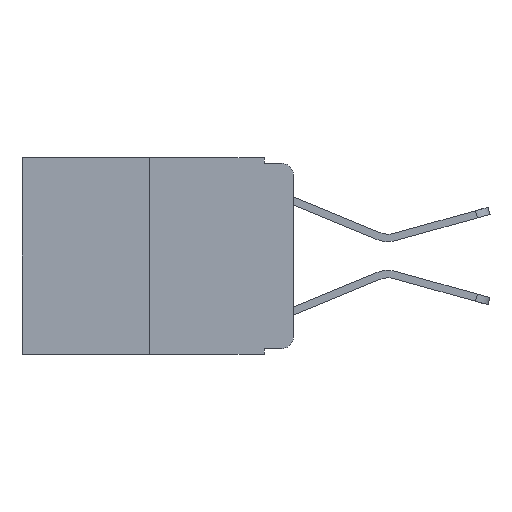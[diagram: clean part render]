
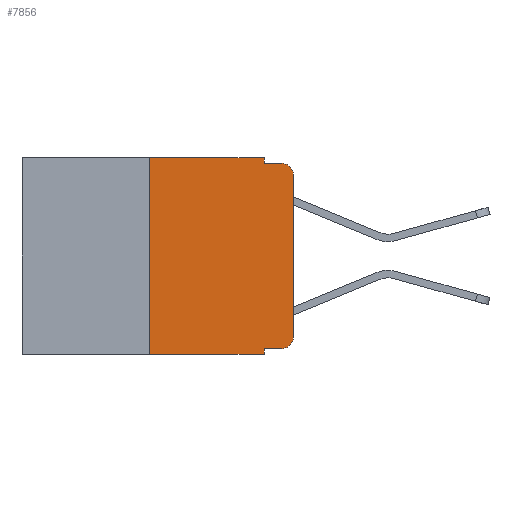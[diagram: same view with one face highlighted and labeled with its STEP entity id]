
A CAD part, left-side view. The second image highlights one B-rep face of the part: STEP entity #7856.
In plain terms, the highlighted planar face has unit normal (-1, 0, 0).
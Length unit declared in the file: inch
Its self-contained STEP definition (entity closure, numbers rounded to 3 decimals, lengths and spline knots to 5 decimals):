
#5 = VERTEX_POINT ( 'NONE', #3871 ) ;
#166 = CARTESIAN_POINT ( 'NONE',  ( 0., 0.25, 0. ) ) ;
#216 = EDGE_CURVE ( 'NONE', #5, #2470, #9156, .T. ) ;
#319 = ORIENTED_EDGE ( 'NONE', *, *, #1063, .F. ) ;
#323 = EDGE_LOOP ( 'NONE', ( #1904, #2161, #2324, #2454, #2485, #7435, #2875, #319, #4257, #5100 ) ) ;
#341 = CARTESIAN_POINT ( 'NONE',  ( 0., 0.25, -0.343 ) ) ;
#346 = VECTOR ( 'NONE', #6810, 39.37008 ) ;
#499 = CARTESIAN_POINT ( 'NONE',  ( 0., 0., -0.03 ) ) ;
#514 = AXIS2_PLACEMENT_3D ( 'NONE', #4303, #12823, #5590 ) ;
#1063 = EDGE_CURVE ( 'NONE', #5, #8498, #13009, .T. ) ;
#1744 = DIRECTION ( 'NONE',  ( 0., -1., 0. ) ) ;
#1848 = CARTESIAN_POINT ( 'NONE',  ( 0., 0.051, 0. ) ) ;
#1904 = ORIENTED_EDGE ( 'NONE', *, *, #8806, .T. ) ;
#1977 = CARTESIAN_POINT ( 'NONE',  ( 0., 0.051, 0. ) ) ;
#2161 = ORIENTED_EDGE ( 'NONE', *, *, #7981, .T. ) ;
#2324 = ORIENTED_EDGE ( 'NONE', *, *, #5486, .F. ) ;
#2404 = VECTOR ( 'NONE', #11945, 39.37008 ) ;
#2454 = ORIENTED_EDGE ( 'NONE', *, *, #3741, .F. ) ;
#2470 = VERTEX_POINT ( 'NONE', #2693 ) ;
#2485 = ORIENTED_EDGE ( 'NONE', *, *, #15749, .F. ) ;
#2685 = VERTEX_POINT ( 'NONE', #341 ) ;
#2693 = CARTESIAN_POINT ( 'NONE',  ( 0., 0.02, -0.333 ) ) ;
#2694 = LINE ( 'NONE', #12845, #12187 ) ;
#2860 = EDGE_CURVE ( 'NONE', #2685, #3075, #4385, .T. ) ;
#2875 = ORIENTED_EDGE ( 'NONE', *, *, #8197, .T. ) ;
#2983 = CARTESIAN_POINT ( 'NONE',  ( 0., 0.051, -0.01 ) ) ;
#3075 = VERTEX_POINT ( 'NONE', #166 ) ;
#3211 = VECTOR ( 'NONE', #13845, 39.37008 ) ;
#3701 = CARTESIAN_POINT ( 'NONE',  ( 0., 0.051, -0.343 ) ) ;
#3741 = EDGE_CURVE ( 'NONE', #4165, #13843, #6296, .T. ) ;
#3871 = CARTESIAN_POINT ( 'NONE',  ( 0., 0.051, -0.333 ) ) ;
#4165 = VERTEX_POINT ( 'NONE', #1848 ) ;
#4257 = ORIENTED_EDGE ( 'NONE', *, *, #216, .T. ) ;
#4303 = CARTESIAN_POINT ( 'NONE',  ( 0., 0.02, -0.313 ) ) ;
#4385 = LINE ( 'NONE', #5404, #13711 ) ;
#4788 = VECTOR ( 'NONE', #1744, 39.37008 ) ;
#4849 = AXIS2_PLACEMENT_3D ( 'NONE', #13296, #7329, #15657 ) ;
#5100 = ORIENTED_EDGE ( 'NONE', *, *, #14660, .T. ) ;
#5351 = CARTESIAN_POINT ( 'NONE',  ( 0., 0.051, -0.333 ) ) ;
#5404 = CARTESIAN_POINT ( 'NONE',  ( 0., 0.25, 0. ) ) ;
#5486 = EDGE_CURVE ( 'NONE', #13843, #7908, #5667, .T. ) ;
#5559 = CARTESIAN_POINT ( 'NONE',  ( 0., 0.473, 0. ) ) ;
#5590 = DIRECTION ( 'NONE',  ( 0., 0., -1. ) ) ;
#5667 = LINE ( 'NONE', #14328, #6063 ) ;
#6063 = VECTOR ( 'NONE', #7159, 39.37008 ) ;
#6294 = CARTESIAN_POINT ( 'NONE',  ( 0., 0.02, -0.03 ) ) ;
#6296 = LINE ( 'NONE', #1977, #15480 ) ;
#6566 = FACE_OUTER_BOUND ( 'NONE', #323, .T. ) ;
#6810 = DIRECTION ( 'NONE',  ( 0., -1., 0. ) ) ;
#7159 = DIRECTION ( 'NONE',  ( 0., -1., 0. ) ) ;
#7329 = DIRECTION ( 'NONE',  ( 1., 0., 0. ) ) ;
#7435 = ORIENTED_EDGE ( 'NONE', *, *, #2860, .F. ) ;
#7530 = DIRECTION ( 'NONE',  ( 0., 0., -1. ) ) ;
#7856 = ADVANCED_FACE ( 'NONE', ( #6566 ), #14434, .F. ) ;
#7908 = VERTEX_POINT ( 'NONE', #9816 ) ;
#7981 = EDGE_CURVE ( 'NONE', #14728, #7908, #11475, .T. ) ;
#8189 = AXIS2_PLACEMENT_3D ( 'NONE', #6294, #14683, #7530 ) ;
#8197 = EDGE_CURVE ( 'NONE', #2685, #8498, #14437, .T. ) ;
#8461 = CARTESIAN_POINT ( 'NONE',  ( 0., 0.051, 0. ) ) ;
#8498 = VERTEX_POINT ( 'NONE', #3701 ) ;
#8806 = EDGE_CURVE ( 'NONE', #13870, #14728, #2694, .T. ) ;
#9156 = LINE ( 'NONE', #5351, #2404 ) ;
#9359 = CARTESIAN_POINT ( 'NONE',  ( 0., 0.473, -0.343 ) ) ;
#9816 = CARTESIAN_POINT ( 'NONE',  ( 0., 0.02, -0.01 ) ) ;
#10735 = DIRECTION ( 'NONE',  ( 0., 0., -1. ) ) ;
#11475 = CIRCLE ( 'NONE', #8189, 0.02 ) ;
#11672 = DIRECTION ( 'NONE',  ( 0., 0., 1. ) ) ;
#11945 = DIRECTION ( 'NONE',  ( 0., -1., 0. ) ) ;
#12187 = VECTOR ( 'NONE', #11672, 39.37008 ) ;
#12823 = DIRECTION ( 'NONE',  ( -1., 0., 0. ) ) ;
#12845 = CARTESIAN_POINT ( 'NONE',  ( 0., 0., 0. ) ) ;
#13009 = LINE ( 'NONE', #8461, #3211 ) ;
#13296 = CARTESIAN_POINT ( 'NONE',  ( 0., 0.473, 0. ) ) ;
#13594 = LINE ( 'NONE', #5559, #346 ) ;
#13711 = VECTOR ( 'NONE', #15291, 39.37008 ) ;
#13843 = VERTEX_POINT ( 'NONE', #2983 ) ;
#13845 = DIRECTION ( 'NONE',  ( 0., 0., -1. ) ) ;
#13870 = VERTEX_POINT ( 'NONE', #15260 ) ;
#14328 = CARTESIAN_POINT ( 'NONE',  ( 0., 0.051, -0.01 ) ) ;
#14434 = PLANE ( 'NONE',  #4849 ) ;
#14437 = LINE ( 'NONE', #9359, #4788 ) ;
#14660 = EDGE_CURVE ( 'NONE', #2470, #13870, #15971, .T. ) ;
#14683 = DIRECTION ( 'NONE',  ( -1., 0., 0. ) ) ;
#14728 = VERTEX_POINT ( 'NONE', #499 ) ;
#15260 = CARTESIAN_POINT ( 'NONE',  ( 0., 0., -0.313 ) ) ;
#15291 = DIRECTION ( 'NONE',  ( 0., 0., 1. ) ) ;
#15480 = VECTOR ( 'NONE', #10735, 39.37008 ) ;
#15657 = DIRECTION ( 'NONE',  ( 0., 0., -1. ) ) ;
#15749 = EDGE_CURVE ( 'NONE', #3075, #4165, #13594, .T. ) ;
#15971 = CIRCLE ( 'NONE', #514, 0.02 ) ;
